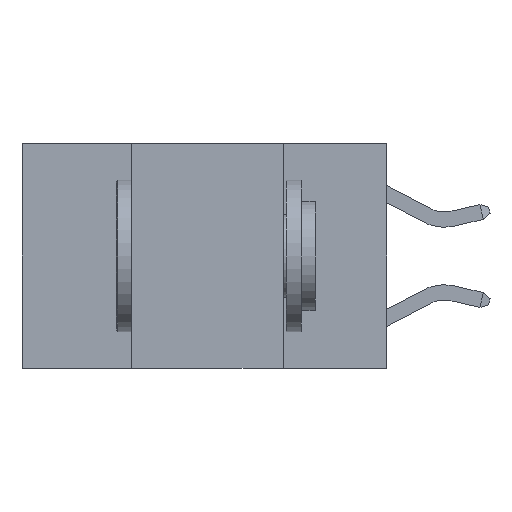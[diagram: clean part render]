
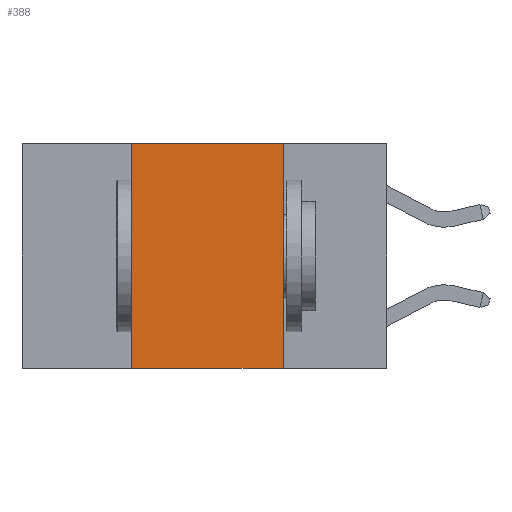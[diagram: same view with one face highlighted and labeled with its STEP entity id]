
A CAD part, left-side view. The second image highlights one B-rep face of the part: STEP entity #388.
In plain terms, the highlighted planar face has unit normal (-1, 0, 0).
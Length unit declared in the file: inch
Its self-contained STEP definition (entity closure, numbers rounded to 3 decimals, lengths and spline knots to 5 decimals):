
#388 = ADVANCED_FACE ( 'NONE', ( #6934 ), #7959, .F. ) ;
#904 = ORIENTED_EDGE ( 'NONE', *, *, #4037, .F. ) ;
#1454 = EDGE_LOOP ( 'NONE', ( #9994, #904, #10112, #3840 ) ) ;
#1672 = EDGE_CURVE ( 'NONE', #7395, #5415, #11468, .T. ) ;
#1829 = EDGE_CURVE ( 'NONE', #7395, #3794, #10194, .T. ) ;
#2489 = DIRECTION ( 'NONE',  ( 0., 0., -1. ) ) ;
#2846 = VECTOR ( 'NONE', #5317, 39.37008 ) ;
#3794 = VERTEX_POINT ( 'NONE', #5227 ) ;
#3834 = EDGE_CURVE ( 'NONE', #7442, #5415, #11557, .T. ) ;
#3840 = ORIENTED_EDGE ( 'NONE', *, *, #1672, .T. ) ;
#4037 = EDGE_CURVE ( 'NONE', #3794, #7442, #9172, .T. ) ;
#4400 = CARTESIAN_POINT ( 'NONE',  ( 0., 0.6, 0. ) ) ;
#4492 = CARTESIAN_POINT ( 'NONE',  ( 0., 0.42, 0. ) ) ;
#5227 = CARTESIAN_POINT ( 'NONE',  ( 0., 0.42, 0. ) ) ;
#5260 = CARTESIAN_POINT ( 'NONE',  ( 0., 0.6, 0. ) ) ;
#5317 = DIRECTION ( 'NONE',  ( 0., -1., 0. ) ) ;
#5415 = VERTEX_POINT ( 'NONE', #11350 ) ;
#6158 = DIRECTION ( 'NONE',  ( 1., 0., 0. ) ) ;
#6297 = VECTOR ( 'NONE', #8078, 39.37008 ) ;
#6934 = FACE_OUTER_BOUND ( 'NONE', #1454, .T. ) ;
#7395 = VERTEX_POINT ( 'NONE', #7996 ) ;
#7442 = VERTEX_POINT ( 'NONE', #9178 ) ;
#7959 = PLANE ( 'NONE',  #9205 ) ;
#7996 = CARTESIAN_POINT ( 'NONE',  ( 0., 0.42, -0.37 ) ) ;
#8078 = DIRECTION ( 'NONE',  ( 0., 0., 1. ) ) ;
#9072 = DIRECTION ( 'NONE',  ( 0., -1., 0. ) ) ;
#9167 = VECTOR ( 'NONE', #2489, 39.37008 ) ;
#9172 = LINE ( 'NONE', #4400, #10322 ) ;
#9178 = CARTESIAN_POINT ( 'NONE',  ( 0., 0.17, 0. ) ) ;
#9205 = AXIS2_PLACEMENT_3D ( 'NONE', #5260, #6158, #9829 ) ;
#9829 = DIRECTION ( 'NONE',  ( 0., 0., -1. ) ) ;
#9994 = ORIENTED_EDGE ( 'NONE', *, *, #3834, .F. ) ;
#10112 = ORIENTED_EDGE ( 'NONE', *, *, #1829, .F. ) ;
#10194 = LINE ( 'NONE', #4492, #6297 ) ;
#10322 = VECTOR ( 'NONE', #9072, 39.37008 ) ;
#10501 = CARTESIAN_POINT ( 'NONE',  ( 0., 0.17, 0. ) ) ;
#10531 = CARTESIAN_POINT ( 'NONE',  ( 0., 0.6, -0.37 ) ) ;
#11350 = CARTESIAN_POINT ( 'NONE',  ( 0., 0.17, -0.37 ) ) ;
#11468 = LINE ( 'NONE', #10531, #2846 ) ;
#11557 = LINE ( 'NONE', #10501, #9167 ) ;
